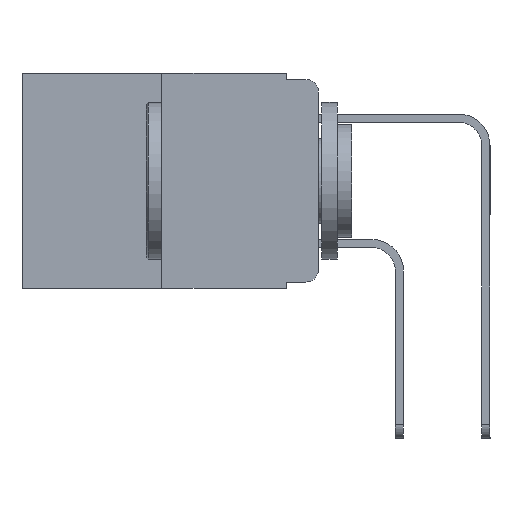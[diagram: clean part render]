
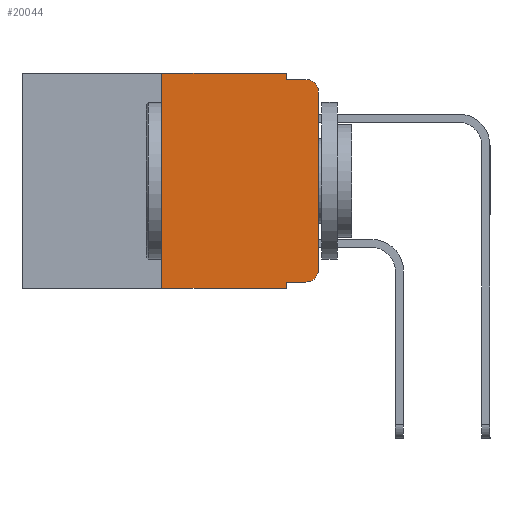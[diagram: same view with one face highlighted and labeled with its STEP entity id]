
A CAD part, left-side view. The second image highlights one B-rep face of the part: STEP entity #20044.
In plain terms, the highlighted planar face has unit normal (-1, 0, 0).
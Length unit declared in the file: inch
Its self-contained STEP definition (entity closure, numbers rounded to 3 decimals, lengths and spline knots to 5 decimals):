
#239 = VERTEX_POINT ( 'NONE', #283 ) ;
#283 = CARTESIAN_POINT ( 'NONE',  ( 0., 0.25, -0.343 ) ) ;
#315 = ORIENTED_EDGE ( 'NONE', *, *, #6468, .F. ) ;
#616 = CARTESIAN_POINT ( 'NONE',  ( 0., 0.051, -0.01 ) ) ;
#756 = DIRECTION ( 'NONE',  ( 0., 0., -1. ) ) ;
#919 = VERTEX_POINT ( 'NONE', #19268 ) ;
#1046 = DIRECTION ( 'NONE',  ( 0., 0., 1. ) ) ;
#1562 = VERTEX_POINT ( 'NONE', #1977 ) ;
#1977 = CARTESIAN_POINT ( 'NONE',  ( 0., 0., -0.313 ) ) ;
#2130 = LINE ( 'NONE', #2509, #6641 ) ;
#2243 = ORIENTED_EDGE ( 'NONE', *, *, #18150, .F. ) ;
#2401 = DIRECTION ( 'NONE',  ( 0., 0., 1. ) ) ;
#2509 = CARTESIAN_POINT ( 'NONE',  ( 0., 0.051, 0. ) ) ;
#2523 = LINE ( 'NONE', #11993, #6511 ) ;
#2558 = DIRECTION ( 'NONE',  ( -1., 0., 0. ) ) ;
#2643 = VECTOR ( 'NONE', #2401, 39.37008 ) ;
#2827 = CARTESIAN_POINT ( 'NONE',  ( 0., 0.02, -0.333 ) ) ;
#3041 = VERTEX_POINT ( 'NONE', #3574 ) ;
#3048 = EDGE_CURVE ( 'NONE', #19480, #12362, #2523, .T. ) ;
#3183 = LINE ( 'NONE', #19128, #12233 ) ;
#3328 = FACE_OUTER_BOUND ( 'NONE', #9187, .T. ) ;
#3465 = DIRECTION ( 'NONE',  ( 1., 0., 0. ) ) ;
#3574 = CARTESIAN_POINT ( 'NONE',  ( 0., 0.02, -0.01 ) ) ;
#3847 = DIRECTION ( 'NONE',  ( 0., 0., -1. ) ) ;
#4207 = CARTESIAN_POINT ( 'NONE',  ( 0., 0.051, -0.333 ) ) ;
#5199 = CARTESIAN_POINT ( 'NONE',  ( 0., 0.473, 0. ) ) ;
#5449 = ORIENTED_EDGE ( 'NONE', *, *, #3048, .T. ) ;
#5952 = DIRECTION ( 'NONE',  ( 0., -1., 0. ) ) ;
#6064 = DIRECTION ( 'NONE',  ( -1., 0., 0. ) ) ;
#6468 = EDGE_CURVE ( 'NONE', #19480, #919, #2130, .T. ) ;
#6501 = CIRCLE ( 'NONE', #8734, 0.02 ) ;
#6511 = VECTOR ( 'NONE', #5952, 39.37008 ) ;
#6641 = VECTOR ( 'NONE', #756, 39.37008 ) ;
#7057 = LINE ( 'NONE', #14012, #11599 ) ;
#7531 = CARTESIAN_POINT ( 'NONE',  ( 0., 0., 0. ) ) ;
#7626 = EDGE_CURVE ( 'NONE', #239, #7891, #20734, .T. ) ;
#7891 = VERTEX_POINT ( 'NONE', #8477 ) ;
#7994 = AXIS2_PLACEMENT_3D ( 'NONE', #13627, #3465, #15278 ) ;
#8394 = ORIENTED_EDGE ( 'NONE', *, *, #13170, .T. ) ;
#8477 = CARTESIAN_POINT ( 'NONE',  ( 0., 0.25, 0. ) ) ;
#8664 = ORIENTED_EDGE ( 'NONE', *, *, #17725, .T. ) ;
#8715 = DIRECTION ( 'NONE',  ( 0., -1., 0. ) ) ;
#8734 = AXIS2_PLACEMENT_3D ( 'NONE', #12751, #2558, #14416 ) ;
#9187 = EDGE_LOOP ( 'NONE', ( #8664, #13663, #18039, #10221, #2243, #20629, #8394, #315, #5449, #14452 ) ) ;
#9344 = VERTEX_POINT ( 'NONE', #17353 ) ;
#9545 = VECTOR ( 'NONE', #8715, 39.37008 ) ;
#9901 = EDGE_CURVE ( 'NONE', #9344, #12155, #7057, .T. ) ;
#10183 = CARTESIAN_POINT ( 'NONE',  ( 0., 0.25, 0. ) ) ;
#10221 = ORIENTED_EDGE ( 'NONE', *, *, #9901, .F. ) ;
#11164 = LINE ( 'NONE', #5199, #19432 ) ;
#11425 = VERTEX_POINT ( 'NONE', #12167 ) ;
#11599 = VECTOR ( 'NONE', #3847, 39.37008 ) ;
#11993 = CARTESIAN_POINT ( 'NONE',  ( 0., 0.051, -0.333 ) ) ;
#12052 = DIRECTION ( 'NONE',  ( 0., -1., 0. ) ) ;
#12155 = VERTEX_POINT ( 'NONE', #616 ) ;
#12167 = CARTESIAN_POINT ( 'NONE',  ( 0., 0., -0.03 ) ) ;
#12181 = EDGE_CURVE ( 'NONE', #12155, #3041, #3183, .T. ) ;
#12233 = VECTOR ( 'NONE', #15912, 39.37008 ) ;
#12362 = VERTEX_POINT ( 'NONE', #2827 ) ;
#12751 = CARTESIAN_POINT ( 'NONE',  ( 0., 0.02, -0.313 ) ) ;
#13170 = EDGE_CURVE ( 'NONE', #239, #919, #14017, .T. ) ;
#13627 = CARTESIAN_POINT ( 'NONE',  ( 0., 0.473, 0. ) ) ;
#13663 = ORIENTED_EDGE ( 'NONE', *, *, #15506, .T. ) ;
#13708 = CARTESIAN_POINT ( 'NONE',  ( 0., 0.473, -0.343 ) ) ;
#14012 = CARTESIAN_POINT ( 'NONE',  ( 0., 0.051, 0. ) ) ;
#14017 = LINE ( 'NONE', #13708, #9545 ) ;
#14416 = DIRECTION ( 'NONE',  ( 0., 0., -1. ) ) ;
#14452 = ORIENTED_EDGE ( 'NONE', *, *, #20344, .T. ) ;
#15278 = DIRECTION ( 'NONE',  ( 0., 0., -1. ) ) ;
#15305 = VECTOR ( 'NONE', #1046, 39.37008 ) ;
#15506 = EDGE_CURVE ( 'NONE', #11425, #3041, #18810, .T. ) ;
#15597 = LINE ( 'NONE', #7531, #2643 ) ;
#15912 = DIRECTION ( 'NONE',  ( 0., -1., 0. ) ) ;
#16171 = CARTESIAN_POINT ( 'NONE',  ( 0., 0.02, -0.03 ) ) ;
#17353 = CARTESIAN_POINT ( 'NONE',  ( 0., 0.051, 0. ) ) ;
#17725 = EDGE_CURVE ( 'NONE', #1562, #11425, #15597, .T. ) ;
#17804 = DIRECTION ( 'NONE',  ( 0., 0., -1. ) ) ;
#18039 = ORIENTED_EDGE ( 'NONE', *, *, #12181, .F. ) ;
#18150 = EDGE_CURVE ( 'NONE', #7891, #9344, #11164, .T. ) ;
#18810 = CIRCLE ( 'NONE', #20337, 0.02 ) ;
#19128 = CARTESIAN_POINT ( 'NONE',  ( 0., 0.051, -0.01 ) ) ;
#19268 = CARTESIAN_POINT ( 'NONE',  ( 0., 0.051, -0.343 ) ) ;
#19432 = VECTOR ( 'NONE', #12052, 39.37008 ) ;
#19480 = VERTEX_POINT ( 'NONE', #4207 ) ;
#20044 = ADVANCED_FACE ( 'NONE', ( #3328 ), #21768, .F. ) ;
#20337 = AXIS2_PLACEMENT_3D ( 'NONE', #16171, #6064, #17804 ) ;
#20344 = EDGE_CURVE ( 'NONE', #12362, #1562, #6501, .T. ) ;
#20629 = ORIENTED_EDGE ( 'NONE', *, *, #7626, .F. ) ;
#20734 = LINE ( 'NONE', #10183, #15305 ) ;
#21768 = PLANE ( 'NONE',  #7994 ) ;
